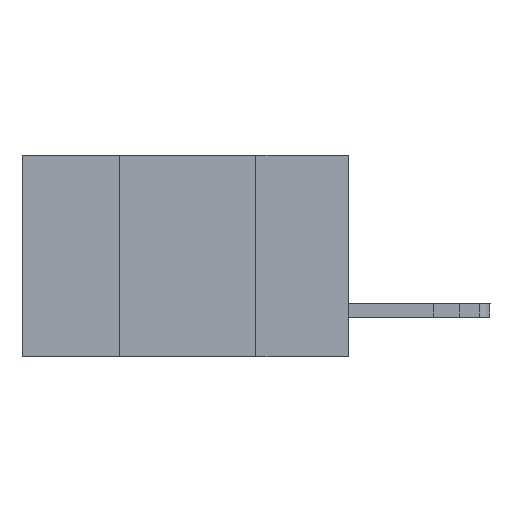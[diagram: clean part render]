
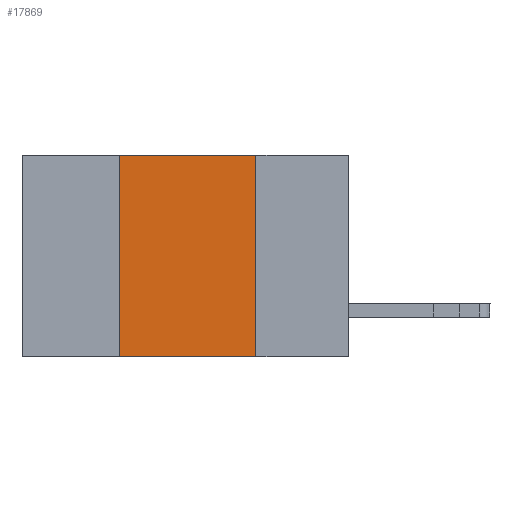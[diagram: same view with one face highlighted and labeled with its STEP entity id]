
A CAD part, left-side view. The second image highlights one B-rep face of the part: STEP entity #17869.
In plain terms, the highlighted planar face has unit normal (-1, 0, 0).
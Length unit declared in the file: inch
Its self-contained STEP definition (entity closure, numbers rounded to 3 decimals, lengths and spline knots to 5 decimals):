
#72 = CARTESIAN_POINT ( 'NONE',  ( 0., 0.42, 0. ) ) ;
#1268 = DIRECTION ( 'NONE',  ( 0., 0., -1. ) ) ;
#1435 = DIRECTION ( 'NONE',  ( 0., 0., 1. ) ) ;
#1535 = CARTESIAN_POINT ( 'NONE',  ( 0., 0.42, -0.37 ) ) ;
#1558 = EDGE_LOOP ( 'NONE', ( #16336, #14470, #14643, #7425 ) ) ;
#1743 = VECTOR ( 'NONE', #4754, 39.37008 ) ;
#2345 = LINE ( 'NONE', #2824, #17139 ) ;
#2824 = CARTESIAN_POINT ( 'NONE',  ( 0., 0.17, -0.37 ) ) ;
#4300 = VERTEX_POINT ( 'NONE', #6378 ) ;
#4754 = DIRECTION ( 'NONE',  ( 0., -1., 0. ) ) ;
#5223 = LINE ( 'NONE', #11911, #13122 ) ;
#5224 = FACE_OUTER_BOUND ( 'NONE', #1558, .T. ) ;
#5632 = EDGE_CURVE ( 'NONE', #7471, #10518, #5223, .T. ) ;
#6378 = CARTESIAN_POINT ( 'NONE',  ( 0., 0.42, -0.37 ) ) ;
#7021 = VECTOR ( 'NONE', #1435, 39.37008 ) ;
#7026 = AXIS2_PLACEMENT_3D ( 'NONE', #7117, #10250, #1268 ) ;
#7117 = CARTESIAN_POINT ( 'NONE',  ( 0., 0.6, 0. ) ) ;
#7258 = EDGE_CURVE ( 'NONE', #4300, #7471, #14882, .T. ) ;
#7425 = ORIENTED_EDGE ( 'NONE', *, *, #15909, .T. ) ;
#7471 = VERTEX_POINT ( 'NONE', #72 ) ;
#10250 = DIRECTION ( 'NONE',  ( 1., 0., 0. ) ) ;
#10518 = VERTEX_POINT ( 'NONE', #17193 ) ;
#11911 = CARTESIAN_POINT ( 'NONE',  ( 0., 0.6, 0. ) ) ;
#12132 = VERTEX_POINT ( 'NONE', #13722 ) ;
#13122 = VECTOR ( 'NONE', #13295, 39.37008 ) ;
#13295 = DIRECTION ( 'NONE',  ( 0., -1., 0. ) ) ;
#13644 = LINE ( 'NONE', #17952, #1743 ) ;
#13722 = CARTESIAN_POINT ( 'NONE',  ( 0., 0.17, -0.37 ) ) ;
#14470 = ORIENTED_EDGE ( 'NONE', *, *, #5632, .F. ) ;
#14643 = ORIENTED_EDGE ( 'NONE', *, *, #7258, .F. ) ;
#14882 = LINE ( 'NONE', #1535, #7021 ) ;
#15045 = EDGE_CURVE ( 'NONE', #10518, #12132, #2345, .T. ) ;
#15909 = EDGE_CURVE ( 'NONE', #4300, #12132, #13644, .T. ) ;
#16336 = ORIENTED_EDGE ( 'NONE', *, *, #15045, .F. ) ;
#17139 = VECTOR ( 'NONE', #17607, 39.37008 ) ;
#17193 = CARTESIAN_POINT ( 'NONE',  ( 0., 0.17, 0. ) ) ;
#17607 = DIRECTION ( 'NONE',  ( 0., 0., -1. ) ) ;
#17869 = ADVANCED_FACE ( 'NONE', ( #5224 ), #18993, .F. ) ;
#17952 = CARTESIAN_POINT ( 'NONE',  ( 0., 0.6, -0.37 ) ) ;
#18993 = PLANE ( 'NONE',  #7026 ) ;
